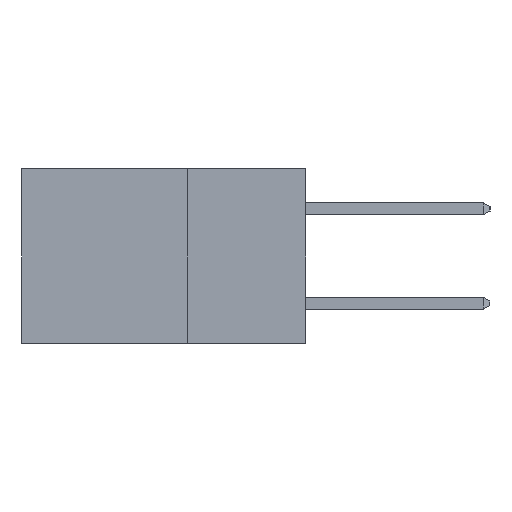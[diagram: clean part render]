
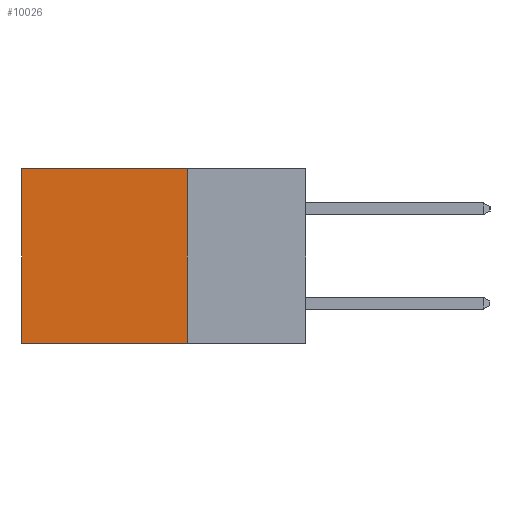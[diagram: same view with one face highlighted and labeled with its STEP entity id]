
A CAD part, left-side view. The second image highlights one B-rep face of the part: STEP entity #10026.
In plain terms, the highlighted planar face has unit normal (-1, 0, 0).
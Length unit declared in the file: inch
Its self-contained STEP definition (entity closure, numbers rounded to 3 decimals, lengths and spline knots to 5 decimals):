
#93 = VERTEX_POINT ( 'NONE', #19522 ) ;
#919 = ORIENTED_EDGE ( 'NONE', *, *, #7406, .T. ) ;
#1404 = AXIS2_PLACEMENT_3D ( 'NONE', #12117, #3187, #1495 ) ;
#1485 = DIRECTION ( 'NONE',  ( 0., 0., -1. ) ) ;
#1495 = DIRECTION ( 'NONE',  ( 0., 0., -1. ) ) ;
#2157 = LINE ( 'NONE', #8940, #23785 ) ;
#2407 = EDGE_LOOP ( 'NONE', ( #919, #23179, #24074, #14939 ) ) ;
#3187 = DIRECTION ( 'NONE',  ( 1., 0., 0. ) ) ;
#3718 = VECTOR ( 'NONE', #15269, 39.37008 ) ;
#4331 = CARTESIAN_POINT ( 'NONE',  ( 0.2615, 0.25, 0. ) ) ;
#5422 = EDGE_CURVE ( 'NONE', #10477, #93, #21232, .T. ) ;
#7049 = CARTESIAN_POINT ( 'NONE',  ( 0.2615, 0.6, -0.37 ) ) ;
#7406 = EDGE_CURVE ( 'NONE', #16345, #18279, #19075, .T. ) ;
#7716 = CARTESIAN_POINT ( 'NONE',  ( 0.2615, 0.25, 0. ) ) ;
#7804 = CARTESIAN_POINT ( 'NONE',  ( 0.2615, 0.6, 0. ) ) ;
#7850 = VECTOR ( 'NONE', #1485, 39.37008 ) ;
#8396 = EDGE_CURVE ( 'NONE', #10477, #16345, #23489, .T. ) ;
#8701 = VECTOR ( 'NONE', #9645, 39.37008 ) ;
#8940 = CARTESIAN_POINT ( 'NONE',  ( 0.2615, 0.25, -0.37 ) ) ;
#9645 = DIRECTION ( 'NONE',  ( 0., 1., 0. ) ) ;
#10026 = ADVANCED_FACE ( 'NONE', ( #16491 ), #24401, .F. ) ;
#10477 = VERTEX_POINT ( 'NONE', #4331 ) ;
#12117 = CARTESIAN_POINT ( 'NONE',  ( 0.2615, 0.25, -0.37 ) ) ;
#14695 = EDGE_CURVE ( 'NONE', #93, #18279, #2157, .T. ) ;
#14939 = ORIENTED_EDGE ( 'NONE', *, *, #8396, .T. ) ;
#15269 = DIRECTION ( 'NONE',  ( 0., 0., -1. ) ) ;
#16345 = VERTEX_POINT ( 'NONE', #7804 ) ;
#16491 = FACE_OUTER_BOUND ( 'NONE', #2407, .T. ) ;
#16826 = DIRECTION ( 'NONE',  ( 0., 1., 0. ) ) ;
#18279 = VERTEX_POINT ( 'NONE', #21455 ) ;
#18664 = CARTESIAN_POINT ( 'NONE',  ( 0.2615, 0.25, -0.37 ) ) ;
#19075 = LINE ( 'NONE', #7049, #7850 ) ;
#19522 = CARTESIAN_POINT ( 'NONE',  ( 0.2615, 0.25, -0.37 ) ) ;
#21232 = LINE ( 'NONE', #18664, #3718 ) ;
#21455 = CARTESIAN_POINT ( 'NONE',  ( 0.2615, 0.6, -0.37 ) ) ;
#23179 = ORIENTED_EDGE ( 'NONE', *, *, #14695, .F. ) ;
#23489 = LINE ( 'NONE', #7716, #8701 ) ;
#23785 = VECTOR ( 'NONE', #16826, 39.37008 ) ;
#24074 = ORIENTED_EDGE ( 'NONE', *, *, #5422, .F. ) ;
#24401 = PLANE ( 'NONE',  #1404 ) ;
